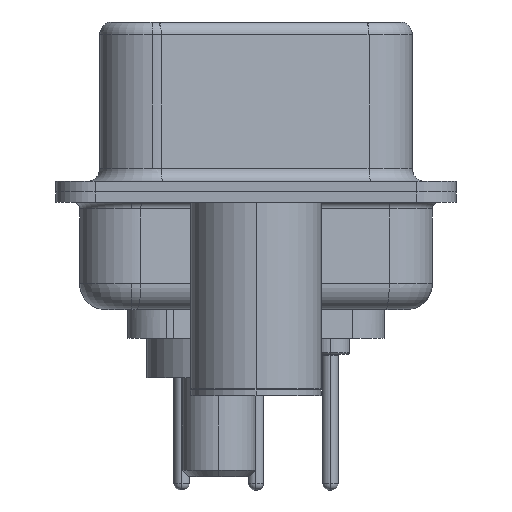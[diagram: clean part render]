
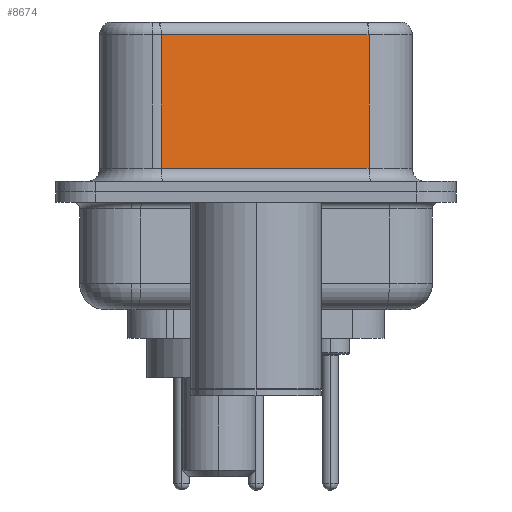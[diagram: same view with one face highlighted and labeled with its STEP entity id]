
A CAD part, left-side view. The second image highlights one B-rep face of the part: STEP entity #8674.
In plain terms, the highlighted planar face has unit normal (-0.985, -0.174, 0).
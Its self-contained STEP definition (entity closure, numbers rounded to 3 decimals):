
#506 = LINE ( 'NONE', #6123, #5487 ) ;
#1028 = ORIENTED_EDGE ( 'NONE', *, *, #7273, .T. ) ;
#1784 = DIRECTION ( 'NONE',  ( -0.174, 0.985, 0. ) ) ;
#3076 = EDGE_CURVE ( 'NONE', #13719, #9420, #6713, .T. ) ;
#3468 = CARTESIAN_POINT ( 'NONE',  ( 3.73, 3.628, 6.02 ) ) ;
#3663 = CARTESIAN_POINT ( 'NONE',  ( 5.132, -4.322, 6.02 ) ) ;
#4655 = LINE ( 'NONE', #13636, #15002 ) ;
#5487 = VECTOR ( 'NONE', #10194, 1000. ) ;
#6085 = VECTOR ( 'NONE', #20581, 1000. ) ;
#6123 = CARTESIAN_POINT ( 'NONE',  ( 5.132, -4.322, 6.52 ) ) ;
#6713 = LINE ( 'NONE', #17053, #6085 ) ;
#7160 = FACE_OUTER_BOUND ( 'NONE', #24724, .T. ) ;
#7273 = EDGE_CURVE ( 'NONE', #16400, #13719, #4655, .T. ) ;
#8006 = PLANE ( 'NONE',  #11042 ) ;
#8674 = ADVANCED_FACE ( 'NONE', ( #7160 ), #8006, .F. ) ;
#9420 = VERTEX_POINT ( 'NONE', #14468 ) ;
#10019 = DIRECTION ( 'NONE',  ( -0.174, 0.985, 0. ) ) ;
#10050 = EDGE_CURVE ( 'NONE', #17481, #9420, #506, .T. ) ;
#10083 = CARTESIAN_POINT ( 'NONE',  ( 5.132, -4.322, 6.52 ) ) ;
#10194 = DIRECTION ( 'NONE',  ( 0., 0., -1. ) ) ;
#10906 = ORIENTED_EDGE ( 'NONE', *, *, #26415, .T. ) ;
#11042 = AXIS2_PLACEMENT_3D ( 'NONE', #10083, #14219, #1784 ) ;
#12955 = ORIENTED_EDGE ( 'NONE', *, *, #3076, .T. ) ;
#13046 = ORIENTED_EDGE ( 'NONE', *, *, #10050, .F. ) ;
#13636 = CARTESIAN_POINT ( 'NONE',  ( 3.73, 3.628, 6.52 ) ) ;
#13719 = VERTEX_POINT ( 'NONE', #25455 ) ;
#14219 = DIRECTION ( 'NONE',  ( 0.985, 0.174, 0. ) ) ;
#14468 = CARTESIAN_POINT ( 'NONE',  ( 5.132, -4.322, 0.9 ) ) ;
#15002 = VECTOR ( 'NONE', #15726, 1000. ) ;
#15726 = DIRECTION ( 'NONE',  ( 0., 0., -1. ) ) ;
#16400 = VERTEX_POINT ( 'NONE', #3468 ) ;
#17053 = CARTESIAN_POINT ( 'NONE',  ( 5.132, -4.322, 0.9 ) ) ;
#17303 = VECTOR ( 'NONE', #10019, 1000. ) ;
#17481 = VERTEX_POINT ( 'NONE', #21603 ) ;
#19855 = LINE ( 'NONE', #3663, #17303 ) ;
#20581 = DIRECTION ( 'NONE',  ( 0.174, -0.985, 0. ) ) ;
#21603 = CARTESIAN_POINT ( 'NONE',  ( 5.132, -4.322, 6.02 ) ) ;
#24724 = EDGE_LOOP ( 'NONE', ( #13046, #10906, #1028, #12955 ) ) ;
#25455 = CARTESIAN_POINT ( 'NONE',  ( 3.73, 3.628, 0.9 ) ) ;
#26415 = EDGE_CURVE ( 'NONE', #17481, #16400, #19855, .T. ) ;
